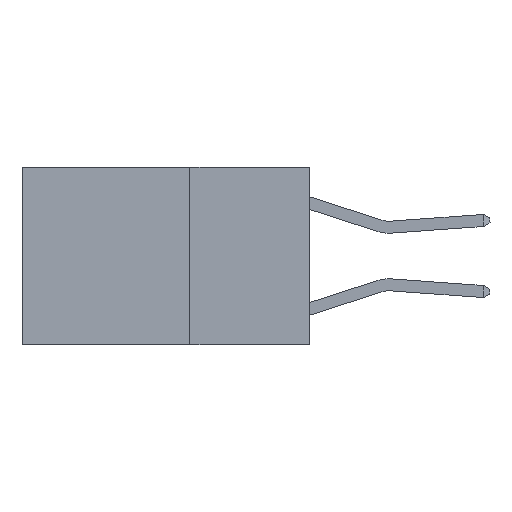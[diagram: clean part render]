
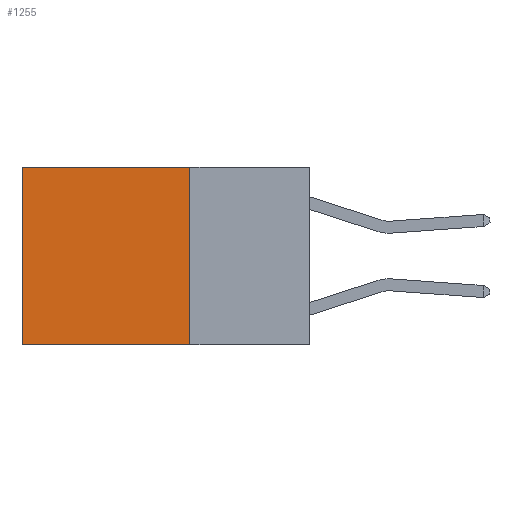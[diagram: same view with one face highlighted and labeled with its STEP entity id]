
A CAD part, left-side view. The second image highlights one B-rep face of the part: STEP entity #1255.
In plain terms, the highlighted planar face has unit normal (-1, 0, 0).
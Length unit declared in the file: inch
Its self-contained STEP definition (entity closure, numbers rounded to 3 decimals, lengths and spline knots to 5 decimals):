
#77 = ORIENTED_EDGE ( 'NONE', *, *, #6601, .T. ) ;
#1138 = CARTESIAN_POINT ( 'NONE',  ( 0.2625, 0.6, 0. ) ) ;
#1255 = ADVANCED_FACE ( 'NONE', ( #5062 ), #12089, .F. ) ;
#1821 = CARTESIAN_POINT ( 'NONE',  ( 0.2625, 0.25, -0.37 ) ) ;
#1973 = CARTESIAN_POINT ( 'NONE',  ( 0.2625, 0.25, 0. ) ) ;
#2398 = LINE ( 'NONE', #14434, #11741 ) ;
#2402 = VERTEX_POINT ( 'NONE', #1821 ) ;
#2591 = DIRECTION ( 'NONE',  ( 0., 1., 0. ) ) ;
#3111 = ORIENTED_EDGE ( 'NONE', *, *, #13355, .F. ) ;
#3361 = EDGE_LOOP ( 'NONE', ( #77, #3111, #11087, #14716 ) ) ;
#3385 = LINE ( 'NONE', #1138, #4227 ) ;
#3866 = VERTEX_POINT ( 'NONE', #7312 ) ;
#4227 = VECTOR ( 'NONE', #13172, 39.37008 ) ;
#5062 = FACE_OUTER_BOUND ( 'NONE', #3361, .T. ) ;
#5190 = EDGE_CURVE ( 'NONE', #3866, #13560, #2398, .T. ) ;
#5488 = CARTESIAN_POINT ( 'NONE',  ( 0.2625, 0.25, 0. ) ) ;
#6601 = EDGE_CURVE ( 'NONE', #13560, #8793, #3385, .T. ) ;
#6716 = CARTESIAN_POINT ( 'NONE',  ( 0.2625, 0.6, 0. ) ) ;
#7312 = CARTESIAN_POINT ( 'NONE',  ( 0.2625, 0.25, 0. ) ) ;
#8241 = DIRECTION ( 'NONE',  ( 1., 0., 0. ) ) ;
#8324 = EDGE_CURVE ( 'NONE', #3866, #2402, #10814, .T. ) ;
#8389 = CARTESIAN_POINT ( 'NONE',  ( 0.2625, 0.6, -0.37 ) ) ;
#8529 = DIRECTION ( 'NONE',  ( 0., 0., -1. ) ) ;
#8793 = VERTEX_POINT ( 'NONE', #8389 ) ;
#10588 = VECTOR ( 'NONE', #14213, 39.37008 ) ;
#10651 = AXIS2_PLACEMENT_3D ( 'NONE', #5488, #8241, #14770 ) ;
#10814 = LINE ( 'NONE', #1973, #14962 ) ;
#11087 = ORIENTED_EDGE ( 'NONE', *, *, #8324, .F. ) ;
#11741 = VECTOR ( 'NONE', #2591, 39.37008 ) ;
#12089 = PLANE ( 'NONE',  #10651 ) ;
#12401 = LINE ( 'NONE', #16900, #10588 ) ;
#13172 = DIRECTION ( 'NONE',  ( 0., 0., -1. ) ) ;
#13355 = EDGE_CURVE ( 'NONE', #2402, #8793, #12401, .T. ) ;
#13560 = VERTEX_POINT ( 'NONE', #6716 ) ;
#14213 = DIRECTION ( 'NONE',  ( 0., 1., 0. ) ) ;
#14434 = CARTESIAN_POINT ( 'NONE',  ( 0.2625, 0.25, 0. ) ) ;
#14716 = ORIENTED_EDGE ( 'NONE', *, *, #5190, .T. ) ;
#14770 = DIRECTION ( 'NONE',  ( 0., 0., -1. ) ) ;
#14962 = VECTOR ( 'NONE', #8529, 39.37008 ) ;
#16900 = CARTESIAN_POINT ( 'NONE',  ( 0.2625, 0.25, -0.37 ) ) ;
